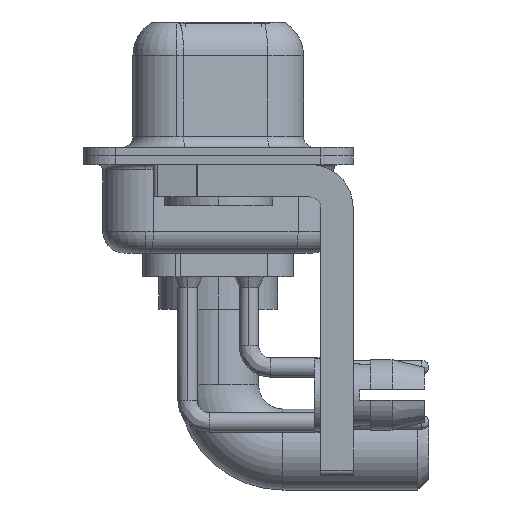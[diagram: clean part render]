
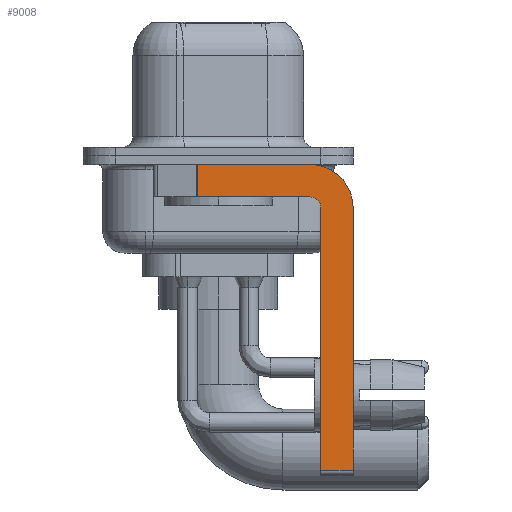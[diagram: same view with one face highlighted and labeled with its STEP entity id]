
A CAD part, left-side view. The second image highlights one B-rep face of the part: STEP entity #9008.
In plain terms, the highlighted planar face has unit normal (-1, 0, 0).
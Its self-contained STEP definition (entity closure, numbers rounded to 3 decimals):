
#1082 = ORIENTED_EDGE ( 'NONE', *, *, #21122, .F. ) ;
#1411 = LINE ( 'NONE', #3295, #22401 ) ;
#1791 = CARTESIAN_POINT ( 'NONE',  ( -2.9, -4.25, -2.4 ) ) ;
#2234 = VERTEX_POINT ( 'NONE', #8540 ) ;
#2566 = CARTESIAN_POINT ( 'NONE',  ( -2.9, -4.25, -1.9 ) ) ;
#2686 = LINE ( 'NONE', #2566, #24318 ) ;
#3032 = CARTESIAN_POINT ( 'NONE',  ( -2.9, 3., -0.4 ) ) ;
#3295 = CARTESIAN_POINT ( 'NONE',  ( -2.9, -4.75, -14.8 ) ) ;
#3575 = EDGE_CURVE ( 'NONE', #13242, #2234, #23720, .T. ) ;
#3837 = EDGE_LOOP ( 'NONE', ( #15027, #13331, #16194, #22366, #22732, #17122, #1082, #18044 ) ) ;
#4357 = DIRECTION ( 'NONE',  ( -1., 0., 0. ) ) ;
#4669 = VERTEX_POINT ( 'NONE', #4867 ) ;
#4678 = DIRECTION ( 'NONE',  ( 0., -1., 0. ) ) ;
#4867 = CARTESIAN_POINT ( 'NONE',  ( -2.9, -4.25, -1.9 ) ) ;
#5460 = VECTOR ( 'NONE', #17656, 1000. ) ;
#5954 = EDGE_CURVE ( 'NONE', #14692, #24477, #24172, .T. ) ;
#6556 = CARTESIAN_POINT ( 'NONE',  ( -2.9, -6.25, -2.4 ) ) ;
#6559 = CARTESIAN_POINT ( 'NONE',  ( -2.9, 0.978, -1.9 ) ) ;
#7289 = PLANE ( 'NONE',  #11117 ) ;
#7609 = DIRECTION ( 'NONE',  ( 0., 0., 1. ) ) ;
#7623 = CARTESIAN_POINT ( 'NONE',  ( -2.9, -6.25, -2.4 ) ) ;
#7870 = LINE ( 'NONE', #3032, #10945 ) ;
#8540 = CARTESIAN_POINT ( 'NONE',  ( -2.9, -6.25, -14.55 ) ) ;
#8579 = LINE ( 'NONE', #6556, #24780 ) ;
#8594 = CARTESIAN_POINT ( 'NONE',  ( -2.9, 0.978, -0.4 ) ) ;
#8766 = DIRECTION ( 'NONE',  ( 0., 1., 0. ) ) ;
#8792 = AXIS2_PLACEMENT_3D ( 'NONE', #21345, #4357, #23608 ) ;
#9008 = ADVANCED_FACE ( 'NONE', ( #15299 ), #7289, .F. ) ;
#9317 = CARTESIAN_POINT ( 'NONE',  ( -2.9, -4.25, -2.4 ) ) ;
#9458 = VERTEX_POINT ( 'NONE', #16763 ) ;
#9504 = DIRECTION ( 'NONE',  ( 1., 0., 0. ) ) ;
#9950 = CIRCLE ( 'NONE', #14407, 2. ) ;
#10881 = DIRECTION ( 'NONE',  ( 0., 0., -1. ) ) ;
#10945 = VECTOR ( 'NONE', #4678, 1000. ) ;
#11117 = AXIS2_PLACEMENT_3D ( 'NONE', #9317, #13140, #15170 ) ;
#11666 = CARTESIAN_POINT ( 'NONE',  ( -2.9, 0.978, -1.9 ) ) ;
#11729 = EDGE_CURVE ( 'NONE', #9458, #4669, #14084, .T. ) ;
#13140 = DIRECTION ( 'NONE',  ( 1., 0., 0. ) ) ;
#13242 = VERTEX_POINT ( 'NONE', #14762 ) ;
#13331 = ORIENTED_EDGE ( 'NONE', *, *, #5954, .T. ) ;
#13763 = CARTESIAN_POINT ( 'NONE',  ( -2.9, -4.25, -14.55 ) ) ;
#14032 = VERTEX_POINT ( 'NONE', #7623 ) ;
#14084 = CIRCLE ( 'NONE', #8792, 0.5 ) ;
#14407 = AXIS2_PLACEMENT_3D ( 'NONE', #1791, #9504, #24448 ) ;
#14692 = VERTEX_POINT ( 'NONE', #8594 ) ;
#14762 = CARTESIAN_POINT ( 'NONE',  ( -2.9, -4.75, -14.55 ) ) ;
#14840 = VECTOR ( 'NONE', #18479, 1000. ) ;
#15027 = ORIENTED_EDGE ( 'NONE', *, *, #19239, .F. ) ;
#15170 = DIRECTION ( 'NONE',  ( 0., 0., -1. ) ) ;
#15299 = FACE_OUTER_BOUND ( 'NONE', #3837, .T. ) ;
#16194 = ORIENTED_EDGE ( 'NONE', *, *, #18842, .F. ) ;
#16763 = CARTESIAN_POINT ( 'NONE',  ( -2.9, -4.75, -2.4 ) ) ;
#17122 = ORIENTED_EDGE ( 'NONE', *, *, #3575, .T. ) ;
#17656 = DIRECTION ( 'NONE',  ( 0., -1., 0. ) ) ;
#17865 = VERTEX_POINT ( 'NONE', #23311 ) ;
#18044 = ORIENTED_EDGE ( 'NONE', *, *, #24456, .F. ) ;
#18479 = DIRECTION ( 'NONE',  ( 0., 0., -1. ) ) ;
#18842 = EDGE_CURVE ( 'NONE', #4669, #24477, #2686, .T. ) ;
#19239 = EDGE_CURVE ( 'NONE', #14692, #17865, #7870, .T. ) ;
#21122 = EDGE_CURVE ( 'NONE', #14032, #2234, #8579, .T. ) ;
#21345 = CARTESIAN_POINT ( 'NONE',  ( -2.9, -4.25, -2.4 ) ) ;
#22366 = ORIENTED_EDGE ( 'NONE', *, *, #11729, .F. ) ;
#22401 = VECTOR ( 'NONE', #7609, 1000. ) ;
#22732 = ORIENTED_EDGE ( 'NONE', *, *, #24330, .F. ) ;
#23311 = CARTESIAN_POINT ( 'NONE',  ( -2.9, -4.25, -0.4 ) ) ;
#23608 = DIRECTION ( 'NONE',  ( 0., 0., 1. ) ) ;
#23720 = LINE ( 'NONE', #13763, #5460 ) ;
#24172 = LINE ( 'NONE', #6559, #14840 ) ;
#24318 = VECTOR ( 'NONE', #8766, 1000. ) ;
#24330 = EDGE_CURVE ( 'NONE', #13242, #9458, #1411, .T. ) ;
#24448 = DIRECTION ( 'NONE',  ( 0., 0., -1. ) ) ;
#24456 = EDGE_CURVE ( 'NONE', #17865, #14032, #9950, .T. ) ;
#24477 = VERTEX_POINT ( 'NONE', #11666 ) ;
#24780 = VECTOR ( 'NONE', #10881, 1000. ) ;
